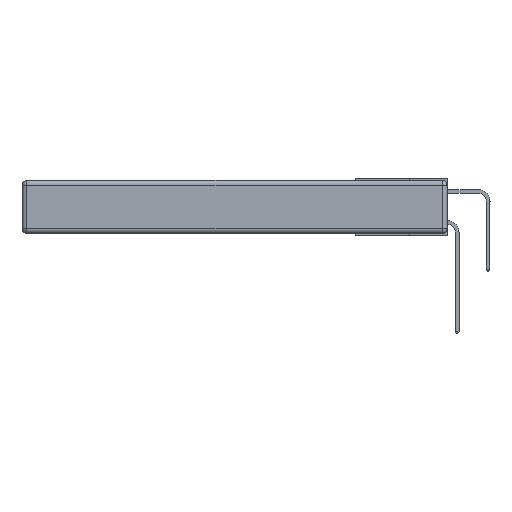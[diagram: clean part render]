
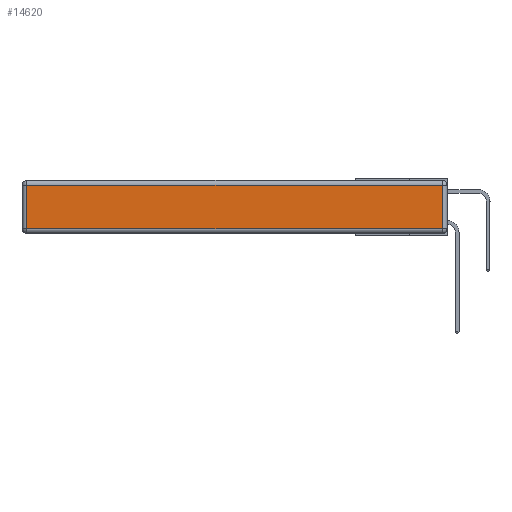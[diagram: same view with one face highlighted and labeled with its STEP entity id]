
A CAD part, left-side view. The second image highlights one B-rep face of the part: STEP entity #14620.
In plain terms, the highlighted planar face has unit normal (-1, 0, 0).
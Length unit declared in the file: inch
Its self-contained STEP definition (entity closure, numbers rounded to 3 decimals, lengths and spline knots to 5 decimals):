
#271 = ORIENTED_EDGE ( 'NONE', *, *, #2194, .T. ) ;
#348 = DIRECTION ( 'NONE',  ( 0., 0., 1. ) ) ;
#1563 = CARTESIAN_POINT ( 'NONE',  ( 0., 0.03, -0.313 ) ) ;
#2194 = EDGE_CURVE ( 'NONE', #11210, #14849, #5046, .T. ) ;
#2575 = CARTESIAN_POINT ( 'NONE',  ( 0., 0.03, -0.03 ) ) ;
#2831 = DIRECTION ( 'NONE',  ( 0., 1., 0. ) ) ;
#3089 = EDGE_CURVE ( 'NONE', #14849, #15078, #14217, .T. ) ;
#3274 = DIRECTION ( 'NONE',  ( 0., -1., 0. ) ) ;
#4233 = AXIS2_PLACEMENT_3D ( 'NONE', #4372, #14609, #14671 ) ;
#4372 = CARTESIAN_POINT ( 'NONE',  ( 0., 0., -0.343 ) ) ;
#5046 = LINE ( 'NONE', #16448, #11503 ) ;
#5094 = EDGE_CURVE ( 'NONE', #9167, #11210, #16972, .T. ) ;
#5198 = ORIENTED_EDGE ( 'NONE', *, *, #16188, .T. ) ;
#5259 = VECTOR ( 'NONE', #11171, 39.37008 ) ;
#6004 = VECTOR ( 'NONE', #2831, 39.37008 ) ;
#9167 = VERTEX_POINT ( 'NONE', #15050 ) ;
#9794 = ORIENTED_EDGE ( 'NONE', *, *, #3089, .T. ) ;
#10228 = CARTESIAN_POINT ( 'NONE',  ( 0., 2.75, -0.03 ) ) ;
#10234 = CARTESIAN_POINT ( 'NONE',  ( 0., 2.72, -0.313 ) ) ;
#11087 = FACE_OUTER_BOUND ( 'NONE', #18426, .T. ) ;
#11171 = DIRECTION ( 'NONE',  ( 0., 0., -1. ) ) ;
#11210 = VERTEX_POINT ( 'NONE', #10234 ) ;
#11503 = VECTOR ( 'NONE', #3274, 39.37008 ) ;
#12594 = CARTESIAN_POINT ( 'NONE',  ( 0., 2.72, -0.343 ) ) ;
#13097 = LINE ( 'NONE', #10228, #6004 ) ;
#13132 = PLANE ( 'NONE',  #4233 ) ;
#13768 = VECTOR ( 'NONE', #348, 39.37008 ) ;
#14217 = LINE ( 'NONE', #15031, #13768 ) ;
#14609 = DIRECTION ( 'NONE',  ( -1., 0., 0. ) ) ;
#14620 = ADVANCED_FACE ( 'NONE', ( #11087 ), #13132, .T. ) ;
#14671 = DIRECTION ( 'NONE',  ( 0., 0., 1. ) ) ;
#14849 = VERTEX_POINT ( 'NONE', #1563 ) ;
#15031 = CARTESIAN_POINT ( 'NONE',  ( 0., 0.03, -0.343 ) ) ;
#15050 = CARTESIAN_POINT ( 'NONE',  ( 0., 2.72, -0.03 ) ) ;
#15078 = VERTEX_POINT ( 'NONE', #2575 ) ;
#15814 = ORIENTED_EDGE ( 'NONE', *, *, #5094, .T. ) ;
#16188 = EDGE_CURVE ( 'NONE', #15078, #9167, #13097, .T. ) ;
#16448 = CARTESIAN_POINT ( 'NONE',  ( 0., 0., -0.313 ) ) ;
#16972 = LINE ( 'NONE', #12594, #5259 ) ;
#18426 = EDGE_LOOP ( 'NONE', ( #271, #9794, #5198, #15814 ) ) ;
